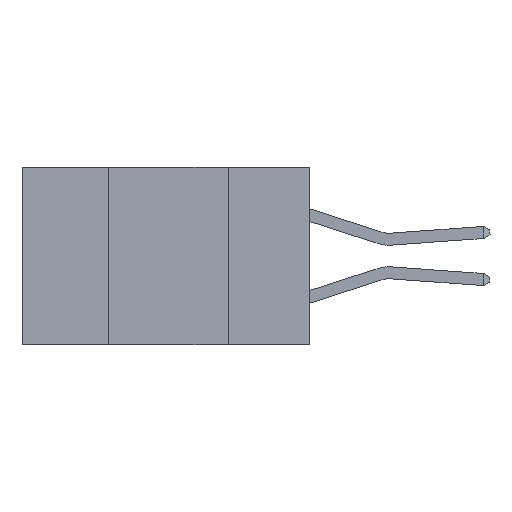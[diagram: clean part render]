
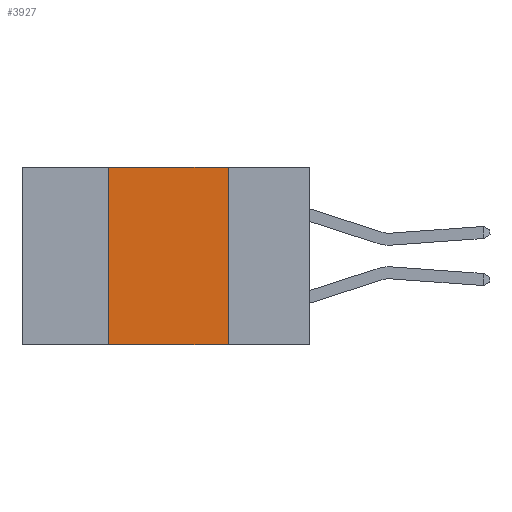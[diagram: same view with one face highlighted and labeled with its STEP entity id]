
A CAD part, left-side view. The second image highlights one B-rep face of the part: STEP entity #3927.
In plain terms, the highlighted planar face has unit normal (-1, 0, 0).
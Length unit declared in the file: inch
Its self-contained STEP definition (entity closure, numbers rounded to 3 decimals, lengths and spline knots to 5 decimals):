
#403 = LINE ( 'NONE', #13088, #8585 ) ;
#741 = ORIENTED_EDGE ( 'NONE', *, *, #5272, .F. ) ;
#1049 = VERTEX_POINT ( 'NONE', #7792 ) ;
#1636 = DIRECTION ( 'NONE',  ( 0., -1., 0. ) ) ;
#1710 = VECTOR ( 'NONE', #1636, 39.37008 ) ;
#1740 = CARTESIAN_POINT ( 'NONE',  ( 0., 0.6, 0. ) ) ;
#1984 = AXIS2_PLACEMENT_3D ( 'NONE', #11437, #11481, #11395 ) ;
#2471 = CARTESIAN_POINT ( 'NONE',  ( 0., 0.17, -0.37 ) ) ;
#2924 = EDGE_LOOP ( 'NONE', ( #4911, #741, #9879, #12470 ) ) ;
#3671 = CARTESIAN_POINT ( 'NONE',  ( 0., 0.42, -0.37 ) ) ;
#3927 = ADVANCED_FACE ( 'NONE', ( #10268 ), #6435, .F. ) ;
#4255 = VERTEX_POINT ( 'NONE', #2471 ) ;
#4305 = CARTESIAN_POINT ( 'NONE',  ( 0., 0.6, -0.37 ) ) ;
#4911 = ORIENTED_EDGE ( 'NONE', *, *, #11637, .F. ) ;
#5200 = DIRECTION ( 'NONE',  ( 0., 0., -1. ) ) ;
#5272 = EDGE_CURVE ( 'NONE', #7396, #1049, #12318, .T. ) ;
#5396 = EDGE_CURVE ( 'NONE', #11273, #7396, #403, .T. ) ;
#5847 = LINE ( 'NONE', #4305, #11019 ) ;
#6099 = CARTESIAN_POINT ( 'NONE',  ( 0., 0.42, 0. ) ) ;
#6435 = PLANE ( 'NONE',  #1984 ) ;
#7310 = LINE ( 'NONE', #9248, #7649 ) ;
#7396 = VERTEX_POINT ( 'NONE', #6099 ) ;
#7649 = VECTOR ( 'NONE', #5200, 39.37008 ) ;
#7792 = CARTESIAN_POINT ( 'NONE',  ( 0., 0.17, 0. ) ) ;
#8417 = DIRECTION ( 'NONE',  ( 0., -1., 0. ) ) ;
#8585 = VECTOR ( 'NONE', #12990, 39.37008 ) ;
#9248 = CARTESIAN_POINT ( 'NONE',  ( 0., 0.17, 0. ) ) ;
#9879 = ORIENTED_EDGE ( 'NONE', *, *, #5396, .F. ) ;
#10268 = FACE_OUTER_BOUND ( 'NONE', #2924, .T. ) ;
#11019 = VECTOR ( 'NONE', #8417, 39.37008 ) ;
#11273 = VERTEX_POINT ( 'NONE', #3671 ) ;
#11395 = DIRECTION ( 'NONE',  ( 0., 0., -1. ) ) ;
#11437 = CARTESIAN_POINT ( 'NONE',  ( 0., 0.6, 0. ) ) ;
#11481 = DIRECTION ( 'NONE',  ( 1., 0., 0. ) ) ;
#11637 = EDGE_CURVE ( 'NONE', #1049, #4255, #7310, .T. ) ;
#12318 = LINE ( 'NONE', #1740, #1710 ) ;
#12384 = EDGE_CURVE ( 'NONE', #11273, #4255, #5847, .T. ) ;
#12470 = ORIENTED_EDGE ( 'NONE', *, *, #12384, .T. ) ;
#12990 = DIRECTION ( 'NONE',  ( 0., 0., 1. ) ) ;
#13088 = CARTESIAN_POINT ( 'NONE',  ( 0., 0.42, 0. ) ) ;
